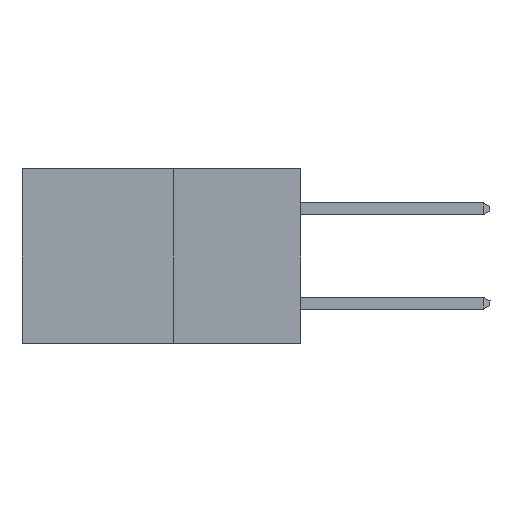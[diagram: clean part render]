
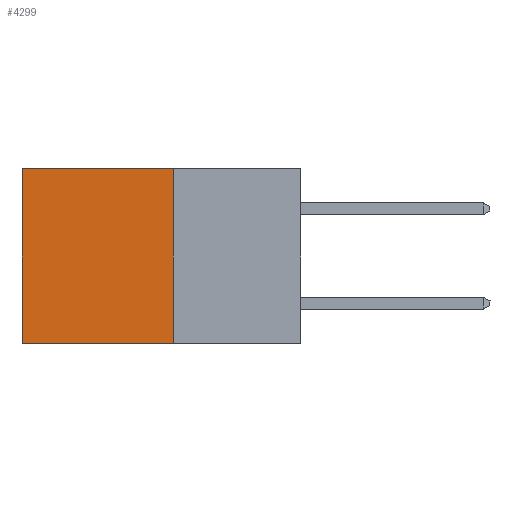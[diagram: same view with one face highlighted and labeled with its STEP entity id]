
A CAD part, left-side view. The second image highlights one B-rep face of the part: STEP entity #4299.
In plain terms, the highlighted planar face has unit normal (-1, 0, 0).
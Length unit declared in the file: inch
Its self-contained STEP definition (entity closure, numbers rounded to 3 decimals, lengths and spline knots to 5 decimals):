
#1702 = EDGE_LOOP ( 'NONE', ( #1995, #15927, #26793, #29116 ) ) ;
#1995 = ORIENTED_EDGE ( 'NONE', *, *, #3701, .T. ) ;
#2691 = VERTEX_POINT ( 'NONE', #10533 ) ;
#3152 = DIRECTION ( 'NONE',  ( 0., 0., -1. ) ) ;
#3632 = CARTESIAN_POINT ( 'NONE',  ( 0.277, 0.27, -0.37 ) ) ;
#3701 = EDGE_CURVE ( 'NONE', #4168, #32922, #26811, .T. ) ;
#4168 = VERTEX_POINT ( 'NONE', #22187 ) ;
#4299 = ADVANCED_FACE ( 'NONE', ( #29613 ), #30257, .F. ) ;
#5429 = DIRECTION ( 'NONE',  ( 1., 0., 0. ) ) ;
#5765 = VECTOR ( 'NONE', #3152, 39.37008 ) ;
#6227 = DIRECTION ( 'NONE',  ( 0., 0., -1. ) ) ;
#6847 = LINE ( 'NONE', #29720, #20078 ) ;
#10533 = CARTESIAN_POINT ( 'NONE',  ( 0.277, 0.27, -0.37 ) ) ;
#11403 = DIRECTION ( 'NONE',  ( 0., 0., -1. ) ) ;
#13520 = CARTESIAN_POINT ( 'NONE',  ( 0.277, 0.59, -0.37 ) ) ;
#15927 = ORIENTED_EDGE ( 'NONE', *, *, #31249, .F. ) ;
#16848 = CARTESIAN_POINT ( 'NONE',  ( 0.277, 0.27, 0. ) ) ;
#17795 = CARTESIAN_POINT ( 'NONE',  ( 0.277, 0.59, -0.37 ) ) ;
#19464 = EDGE_CURVE ( 'NONE', #31245, #4168, #30937, .T. ) ;
#20078 = VECTOR ( 'NONE', #11403, 39.37008 ) ;
#22187 = CARTESIAN_POINT ( 'NONE',  ( 0.277, 0.59, 0. ) ) ;
#22616 = CARTESIAN_POINT ( 'NONE',  ( 0.277, 0.27, 0. ) ) ;
#24052 = VECTOR ( 'NONE', #33021, 39.37008 ) ;
#24405 = AXIS2_PLACEMENT_3D ( 'NONE', #29274, #5429, #6227 ) ;
#24793 = DIRECTION ( 'NONE',  ( 0., 1., 0. ) ) ;
#25223 = LINE ( 'NONE', #3632, #31280 ) ;
#26793 = ORIENTED_EDGE ( 'NONE', *, *, #28484, .F. ) ;
#26811 = LINE ( 'NONE', #17795, #5765 ) ;
#28484 = EDGE_CURVE ( 'NONE', #31245, #2691, #6847, .T. ) ;
#29116 = ORIENTED_EDGE ( 'NONE', *, *, #19464, .T. ) ;
#29274 = CARTESIAN_POINT ( 'NONE',  ( 0.277, 0.27, -0.37 ) ) ;
#29613 = FACE_OUTER_BOUND ( 'NONE', #1702, .T. ) ;
#29720 = CARTESIAN_POINT ( 'NONE',  ( 0.277, 0.27, -0.37 ) ) ;
#30257 = PLANE ( 'NONE',  #24405 ) ;
#30937 = LINE ( 'NONE', #22616, #24052 ) ;
#31245 = VERTEX_POINT ( 'NONE', #16848 ) ;
#31249 = EDGE_CURVE ( 'NONE', #2691, #32922, #25223, .T. ) ;
#31280 = VECTOR ( 'NONE', #24793, 39.37008 ) ;
#32922 = VERTEX_POINT ( 'NONE', #13520 ) ;
#33021 = DIRECTION ( 'NONE',  ( 0., 1., 0. ) ) ;
